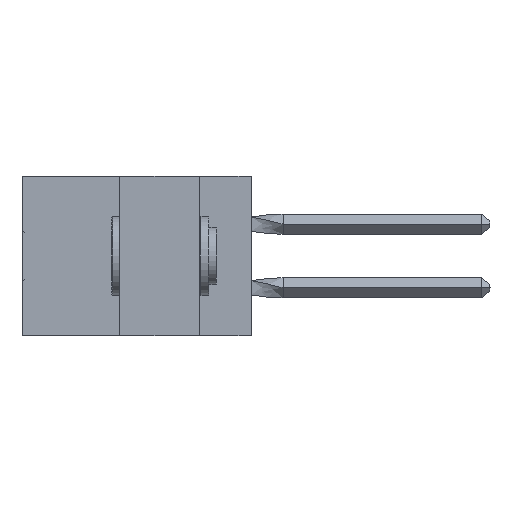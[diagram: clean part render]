
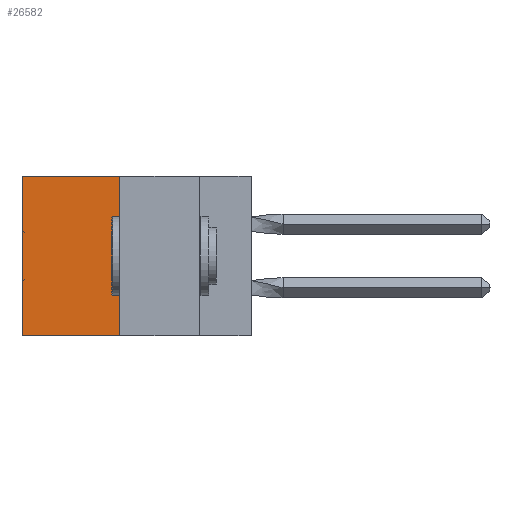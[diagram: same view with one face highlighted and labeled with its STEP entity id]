
A CAD part, left-side view. The second image highlights one B-rep face of the part: STEP entity #26582.
In plain terms, the highlighted planar face has unit normal (-1, 0, 0).
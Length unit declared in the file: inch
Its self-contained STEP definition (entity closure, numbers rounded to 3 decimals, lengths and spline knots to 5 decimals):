
#5473 = EDGE_CURVE ( 'NONE', #35109, #20147, #8084, .T. ) ;
#7432 = VERTEX_POINT ( 'NONE', #12959 ) ;
#8055 = LINE ( 'NONE', #17925, #27187 ) ;
#8084 = LINE ( 'NONE', #17336, #34341 ) ;
#9458 = DIRECTION ( 'NONE',  ( 0., 1., 0. ) ) ;
#10193 = CARTESIAN_POINT ( 'NONE',  ( 0.305, 0.72, -0.5 ) ) ;
#10568 = PLANE ( 'NONE',  #29481 ) ;
#10764 = EDGE_CURVE ( 'NONE', #7432, #20147, #46069, .T. ) ;
#12959 = CARTESIAN_POINT ( 'NONE',  ( 0.305, 0.413, -0.5 ) ) ;
#13485 = DIRECTION ( 'NONE',  ( 0., 0., -1. ) ) ;
#13609 = DIRECTION ( 'NONE',  ( 1., 0., 0. ) ) ;
#14184 = EDGE_CURVE ( 'NONE', #37639, #7432, #29262, .T. ) ;
#16827 = CARTESIAN_POINT ( 'NONE',  ( 0.305, 0.413, -0.5 ) ) ;
#17336 = CARTESIAN_POINT ( 'NONE',  ( 0.305, 0.72, -0.5 ) ) ;
#17925 = CARTESIAN_POINT ( 'NONE',  ( 0.305, 0.413, 0. ) ) ;
#19849 = CARTESIAN_POINT ( 'NONE',  ( 0.305, 0.413, 0. ) ) ;
#20147 = VERTEX_POINT ( 'NONE', #10193 ) ;
#21622 = CARTESIAN_POINT ( 'NONE',  ( 0.305, 0.413, -0.5 ) ) ;
#26582 = ADVANCED_FACE ( 'NONE', ( #43144 ), #10568, .F. ) ;
#27164 = ORIENTED_EDGE ( 'NONE', *, *, #5473, .T. ) ;
#27187 = VECTOR ( 'NONE', #44666, 39.37008 ) ;
#29190 = ORIENTED_EDGE ( 'NONE', *, *, #46332, .T. ) ;
#29262 = LINE ( 'NONE', #37848, #47233 ) ;
#29266 = DIRECTION ( 'NONE',  ( 0., 0., -1. ) ) ;
#29481 = AXIS2_PLACEMENT_3D ( 'NONE', #21622, #13609, #29266 ) ;
#33977 = DIRECTION ( 'NONE',  ( 0., 0., -1. ) ) ;
#34341 = VECTOR ( 'NONE', #13485, 39.37008 ) ;
#35109 = VERTEX_POINT ( 'NONE', #35390 ) ;
#35390 = CARTESIAN_POINT ( 'NONE',  ( 0.305, 0.72, 0. ) ) ;
#36170 = ORIENTED_EDGE ( 'NONE', *, *, #10764, .F. ) ;
#37064 = EDGE_LOOP ( 'NONE', ( #27164, #36170, #44354, #29190 ) ) ;
#37639 = VERTEX_POINT ( 'NONE', #19849 ) ;
#37848 = CARTESIAN_POINT ( 'NONE',  ( 0.305, 0.413, -0.5 ) ) ;
#43144 = FACE_OUTER_BOUND ( 'NONE', #37064, .T. ) ;
#44354 = ORIENTED_EDGE ( 'NONE', *, *, #14184, .F. ) ;
#44666 = DIRECTION ( 'NONE',  ( 0., 1., 0. ) ) ;
#46069 = LINE ( 'NONE', #16827, #49028 ) ;
#46332 = EDGE_CURVE ( 'NONE', #37639, #35109, #8055, .T. ) ;
#47233 = VECTOR ( 'NONE', #33977, 39.37008 ) ;
#49028 = VECTOR ( 'NONE', #9458, 39.37008 ) ;
